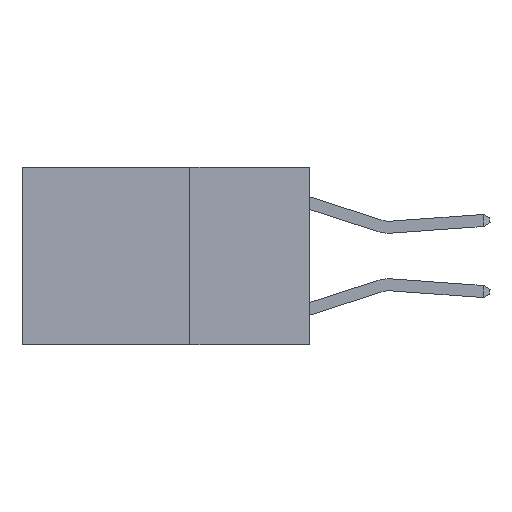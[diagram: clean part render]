
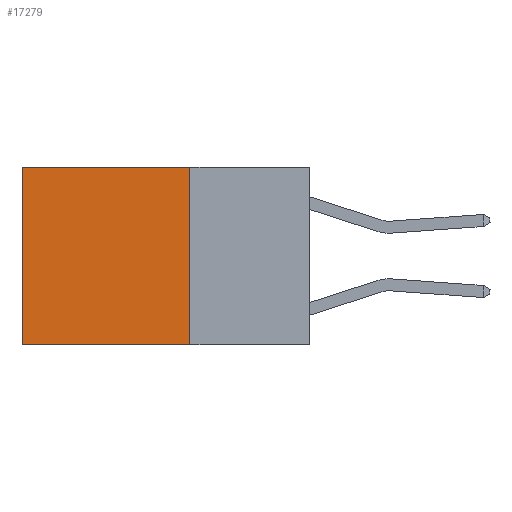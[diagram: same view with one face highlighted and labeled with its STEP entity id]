
A CAD part, left-side view. The second image highlights one B-rep face of the part: STEP entity #17279.
In plain terms, the highlighted planar face has unit normal (-1, 0, 0).
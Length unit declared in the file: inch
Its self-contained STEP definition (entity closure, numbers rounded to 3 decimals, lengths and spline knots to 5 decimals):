
#640 = ORIENTED_EDGE ( 'NONE', *, *, #3988, .F. ) ;
#1163 = CARTESIAN_POINT ( 'NONE',  ( 0.2625, 0.25, -0.37 ) ) ;
#1936 = ORIENTED_EDGE ( 'NONE', *, *, #3485, .T. ) ;
#2033 = VERTEX_POINT ( 'NONE', #9155 ) ;
#2273 = VERTEX_POINT ( 'NONE', #17690 ) ;
#3314 = VECTOR ( 'NONE', #16639, 39.37008 ) ;
#3485 = EDGE_CURVE ( 'NONE', #2273, #13809, #12973, .T. ) ;
#3639 = CARTESIAN_POINT ( 'NONE',  ( 0.2625, 0.6, 0. ) ) ;
#3988 = EDGE_CURVE ( 'NONE', #2273, #2033, #21355, .T. ) ;
#5073 = VECTOR ( 'NONE', #5825, 39.37008 ) ;
#5825 = DIRECTION ( 'NONE',  ( 0., 0., -1. ) ) ;
#7607 = CARTESIAN_POINT ( 'NONE',  ( 0.2625, 0.25, 0. ) ) ;
#9155 = CARTESIAN_POINT ( 'NONE',  ( 0.2625, 0.25, -0.37 ) ) ;
#9156 = DIRECTION ( 'NONE',  ( 0., 1., 0. ) ) ;
#9467 = CARTESIAN_POINT ( 'NONE',  ( 0.2625, 0.6, -0.37 ) ) ;
#9533 = VECTOR ( 'NONE', #9156, 39.37008 ) ;
#12973 = LINE ( 'NONE', #20749, #9533 ) ;
#13342 = ORIENTED_EDGE ( 'NONE', *, *, #15285, .T. ) ;
#13809 = VERTEX_POINT ( 'NONE', #3639 ) ;
#14801 = DIRECTION ( 'NONE',  ( 0., 0., -1. ) ) ;
#15285 = EDGE_CURVE ( 'NONE', #13809, #16952, #22563, .T. ) ;
#15316 = CARTESIAN_POINT ( 'NONE',  ( 0.2625, 0.6, 0. ) ) ;
#16639 = DIRECTION ( 'NONE',  ( 0., 1., 0. ) ) ;
#16952 = VERTEX_POINT ( 'NONE', #9467 ) ;
#17279 = ADVANCED_FACE ( 'NONE', ( #21940 ), #24328, .F. ) ;
#17479 = AXIS2_PLACEMENT_3D ( 'NONE', #23956, #21823, #24207 ) ;
#17690 = CARTESIAN_POINT ( 'NONE',  ( 0.2625, 0.25, 0. ) ) ;
#19330 = ORIENTED_EDGE ( 'NONE', *, *, #19750, .F. ) ;
#19750 = EDGE_CURVE ( 'NONE', #2033, #16952, #20480, .T. ) ;
#20480 = LINE ( 'NONE', #1163, #3314 ) ;
#20749 = CARTESIAN_POINT ( 'NONE',  ( 0.2625, 0.25, 0. ) ) ;
#20759 = EDGE_LOOP ( 'NONE', ( #13342, #19330, #640, #1936 ) ) ;
#21070 = VECTOR ( 'NONE', #14801, 39.37008 ) ;
#21355 = LINE ( 'NONE', #7607, #5073 ) ;
#21823 = DIRECTION ( 'NONE',  ( 1., 0., 0. ) ) ;
#21940 = FACE_OUTER_BOUND ( 'NONE', #20759, .T. ) ;
#22563 = LINE ( 'NONE', #15316, #21070 ) ;
#23956 = CARTESIAN_POINT ( 'NONE',  ( 0.2625, 0.25, 0. ) ) ;
#24207 = DIRECTION ( 'NONE',  ( 0., 0., -1. ) ) ;
#24328 = PLANE ( 'NONE',  #17479 ) ;
